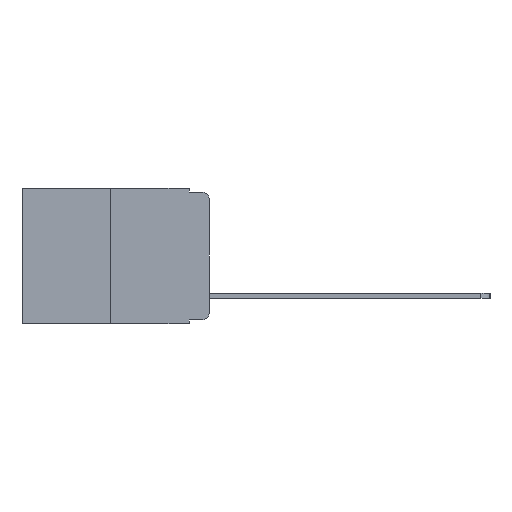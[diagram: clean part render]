
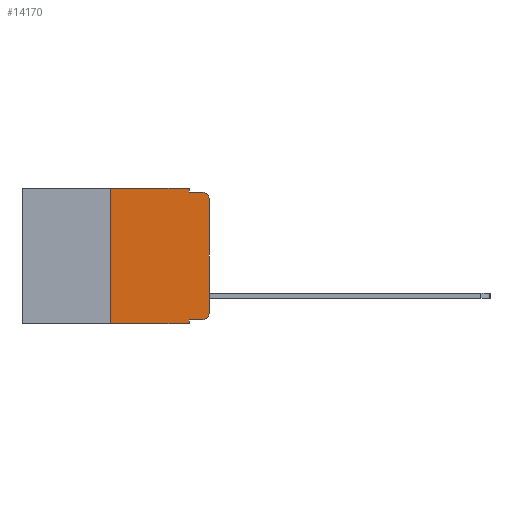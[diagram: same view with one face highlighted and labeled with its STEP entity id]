
A CAD part, left-side view. The second image highlights one B-rep face of the part: STEP entity #14170.
In plain terms, the highlighted planar face has unit normal (-1, 0, 0).
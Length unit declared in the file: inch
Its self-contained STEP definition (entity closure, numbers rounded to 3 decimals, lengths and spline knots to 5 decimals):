
#20 = VERTEX_POINT ( 'NONE', #2743 ) ;
#340 = LINE ( 'NONE', #6336, #18050 ) ;
#490 = DIRECTION ( 'NONE',  ( 0., 0., -1. ) ) ;
#566 = EDGE_CURVE ( 'NONE', #1021, #16944, #13798, .T. ) ;
#738 = CARTESIAN_POINT ( 'NONE',  ( 0., 0.25, -0.343 ) ) ;
#1021 = VERTEX_POINT ( 'NONE', #738 ) ;
#1245 = CARTESIAN_POINT ( 'NONE',  ( 0., 0.02, -0.333 ) ) ;
#1261 = ORIENTED_EDGE ( 'NONE', *, *, #7751, .F. ) ;
#1293 = CIRCLE ( 'NONE', #7014, 0.02 ) ;
#1571 = CARTESIAN_POINT ( 'NONE',  ( 0., 0.25, 0. ) ) ;
#1761 = ORIENTED_EDGE ( 'NONE', *, *, #8163, .T. ) ;
#1839 = LINE ( 'NONE', #14523, #11784 ) ;
#1870 = EDGE_CURVE ( 'NONE', #16944, #11221, #1839, .T. ) ;
#2034 = CARTESIAN_POINT ( 'NONE',  ( 0., 0.473, 0. ) ) ;
#2142 = VECTOR ( 'NONE', #6507, 39.37008 ) ;
#2202 = LINE ( 'NONE', #16589, #12982 ) ;
#2361 = CARTESIAN_POINT ( 'NONE',  ( 0., 0.051, -0.01 ) ) ;
#2617 = LINE ( 'NONE', #2361, #16968 ) ;
#2698 = ORIENTED_EDGE ( 'NONE', *, *, #7210, .T. ) ;
#2743 = CARTESIAN_POINT ( 'NONE',  ( 0., 0., -0.313 ) ) ;
#2809 = ORIENTED_EDGE ( 'NONE', *, *, #13699, .F. ) ;
#3005 = VERTEX_POINT ( 'NONE', #6658 ) ;
#3377 = CARTESIAN_POINT ( 'NONE',  ( 0., 0.051, -0.333 ) ) ;
#4772 = ORIENTED_EDGE ( 'NONE', *, *, #16640, .T. ) ;
#4955 = PLANE ( 'NONE',  #7115 ) ;
#5099 = CARTESIAN_POINT ( 'NONE',  ( 0., 0.051, 0. ) ) ;
#5366 = CARTESIAN_POINT ( 'NONE',  ( 0., 0.02, -0.313 ) ) ;
#5577 = DIRECTION ( 'NONE',  ( -1., 0., 0. ) ) ;
#5980 = LINE ( 'NONE', #5099, #2142 ) ;
#6299 = ORIENTED_EDGE ( 'NONE', *, *, #1870, .F. ) ;
#6300 = ORIENTED_EDGE ( 'NONE', *, *, #10824, .T. ) ;
#6336 = CARTESIAN_POINT ( 'NONE',  ( 0., 0.051, 0. ) ) ;
#6370 = CIRCLE ( 'NONE', #9540, 0.02 ) ;
#6374 = DIRECTION ( 'NONE',  ( 1., 0., 0. ) ) ;
#6410 = VECTOR ( 'NONE', #11677, 39.37008 ) ;
#6470 = DIRECTION ( 'NONE',  ( 0., -1., 0. ) ) ;
#6507 = DIRECTION ( 'NONE',  ( 0., 0., -1. ) ) ;
#6658 = CARTESIAN_POINT ( 'NONE',  ( 0., 0.051, -0.343 ) ) ;
#6773 = DIRECTION ( 'NONE',  ( 0., 0., -1. ) ) ;
#6918 = EDGE_LOOP ( 'NONE', ( #4772, #8304, #11107, #2809, #6299, #10131, #1761, #1261, #6300, #2698 ) ) ;
#6951 = VECTOR ( 'NONE', #12202, 39.37008 ) ;
#7014 = AXIS2_PLACEMENT_3D ( 'NONE', #5366, #15044, #6773 ) ;
#7115 = AXIS2_PLACEMENT_3D ( 'NONE', #2034, #6374, #16014 ) ;
#7136 = VERTEX_POINT ( 'NONE', #14809 ) ;
#7210 = EDGE_CURVE ( 'NONE', #14369, #20, #1293, .T. ) ;
#7751 = EDGE_CURVE ( 'NONE', #7136, #3005, #340, .T. ) ;
#8163 = EDGE_CURVE ( 'NONE', #1021, #3005, #2202, .T. ) ;
#8304 = ORIENTED_EDGE ( 'NONE', *, *, #14353, .T. ) ;
#8729 = CARTESIAN_POINT ( 'NONE',  ( 0., 0.051, 0. ) ) ;
#9374 = DIRECTION ( 'NONE',  ( 0., -1., 0. ) ) ;
#9540 = AXIS2_PLACEMENT_3D ( 'NONE', #13881, #5577, #15242 ) ;
#10131 = ORIENTED_EDGE ( 'NONE', *, *, #566, .F. ) ;
#10452 = EDGE_CURVE ( 'NONE', #15787, #11650, #2617, .T. ) ;
#10824 = EDGE_CURVE ( 'NONE', #7136, #14369, #12267, .T. ) ;
#11107 = ORIENTED_EDGE ( 'NONE', *, *, #10452, .F. ) ;
#11221 = VERTEX_POINT ( 'NONE', #8729 ) ;
#11650 = VERTEX_POINT ( 'NONE', #12343 ) ;
#11677 = DIRECTION ( 'NONE',  ( 0., 0., 1. ) ) ;
#11784 = VECTOR ( 'NONE', #16741, 39.37008 ) ;
#12202 = DIRECTION ( 'NONE',  ( 0., 0., 1. ) ) ;
#12267 = LINE ( 'NONE', #3377, #14199 ) ;
#12343 = CARTESIAN_POINT ( 'NONE',  ( 0., 0.02, -0.01 ) ) ;
#12982 = VECTOR ( 'NONE', #16637, 39.37008 ) ;
#13593 = CARTESIAN_POINT ( 'NONE',  ( 0., 0., 0. ) ) ;
#13699 = EDGE_CURVE ( 'NONE', #11221, #15787, #5980, .T. ) ;
#13798 = LINE ( 'NONE', #1571, #6410 ) ;
#13881 = CARTESIAN_POINT ( 'NONE',  ( 0., 0.02, -0.03 ) ) ;
#14170 = ADVANCED_FACE ( 'NONE', ( #17163 ), #4955, .F. ) ;
#14199 = VECTOR ( 'NONE', #6470, 39.37008 ) ;
#14272 = VERTEX_POINT ( 'NONE', #17671 ) ;
#14353 = EDGE_CURVE ( 'NONE', #14272, #11650, #6370, .T. ) ;
#14369 = VERTEX_POINT ( 'NONE', #1245 ) ;
#14523 = CARTESIAN_POINT ( 'NONE',  ( 0., 0.473, 0. ) ) ;
#14729 = LINE ( 'NONE', #13593, #6951 ) ;
#14809 = CARTESIAN_POINT ( 'NONE',  ( 0., 0.051, -0.333 ) ) ;
#15044 = DIRECTION ( 'NONE',  ( -1., 0., 0. ) ) ;
#15242 = DIRECTION ( 'NONE',  ( 0., 0., -1. ) ) ;
#15633 = CARTESIAN_POINT ( 'NONE',  ( 0., 0.051, -0.01 ) ) ;
#15787 = VERTEX_POINT ( 'NONE', #15633 ) ;
#16014 = DIRECTION ( 'NONE',  ( 0., 0., -1. ) ) ;
#16523 = CARTESIAN_POINT ( 'NONE',  ( 0., 0.25, 0. ) ) ;
#16589 = CARTESIAN_POINT ( 'NONE',  ( 0., 0.473, -0.343 ) ) ;
#16637 = DIRECTION ( 'NONE',  ( 0., -1., 0. ) ) ;
#16640 = EDGE_CURVE ( 'NONE', #20, #14272, #14729, .T. ) ;
#16741 = DIRECTION ( 'NONE',  ( 0., -1., 0. ) ) ;
#16944 = VERTEX_POINT ( 'NONE', #16523 ) ;
#16968 = VECTOR ( 'NONE', #9374, 39.37008 ) ;
#17163 = FACE_OUTER_BOUND ( 'NONE', #6918, .T. ) ;
#17671 = CARTESIAN_POINT ( 'NONE',  ( 0., 0., -0.03 ) ) ;
#18050 = VECTOR ( 'NONE', #490, 39.37008 ) ;
